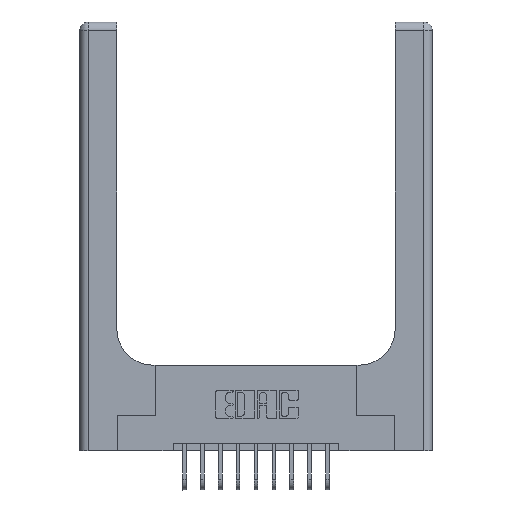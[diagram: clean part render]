
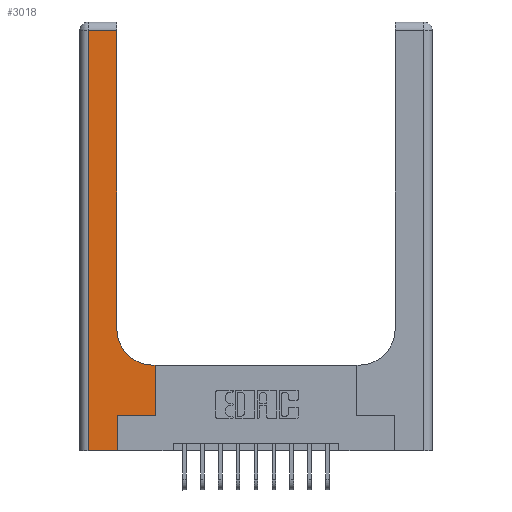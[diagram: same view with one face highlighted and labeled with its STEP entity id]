
A CAD part, top view. The second image highlights one B-rep face of the part: STEP entity #3018.
In plain terms, the highlighted planar face has unit normal (0, 0, 1).
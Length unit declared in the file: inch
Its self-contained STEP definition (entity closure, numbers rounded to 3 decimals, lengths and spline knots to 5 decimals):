
#405 = LINE ( 'NONE', #14723, #9553 ) ;
#573 = DIRECTION ( 'NONE',  ( 0., 0., -1. ) ) ;
#615 = AXIS2_PLACEMENT_3D ( 'NONE', #7003, #573, #727 ) ;
#727 = DIRECTION ( 'NONE',  ( 1., 0., 0. ) ) ;
#802 = DIRECTION ( 'NONE',  ( 0., 0., -1. ) ) ;
#1181 = EDGE_CURVE ( 'NONE', #4048, #1853, #5839, .T. ) ;
#1262 = LINE ( 'NONE', #6699, #10371 ) ;
#1853 = VERTEX_POINT ( 'NONE', #13303 ) ;
#1867 = CARTESIAN_POINT ( 'NONE',  ( 0., 2.94, 0.37 ) ) ;
#1928 = DIRECTION ( 'NONE',  ( 1., 0., 0. ) ) ;
#2001 = EDGE_CURVE ( 'NONE', #9961, #12800, #8169, .T. ) ;
#2038 = VECTOR ( 'NONE', #13661, 39.37008 ) ;
#2502 = EDGE_CURVE ( 'NONE', #14931, #10751, #4890, .T. ) ;
#2544 = ORIENTED_EDGE ( 'NONE', *, *, #8270, .T. ) ;
#2591 = VERTEX_POINT ( 'NONE', #9210 ) ;
#2770 = LINE ( 'NONE', #3832, #11812 ) ;
#3018 = ADVANCED_FACE ( 'NONE', ( #6888 ), #6785, .F. ) ;
#3832 = CARTESIAN_POINT ( 'NONE',  ( 0.06, 3., 0.37 ) ) ;
#4048 = VERTEX_POINT ( 'NONE', #14585 ) ;
#4334 = CARTESIAN_POINT ( 'NONE',  ( 0.265, 0.25, 0.37 ) ) ;
#4401 = VECTOR ( 'NONE', #9011, 39.37008 ) ;
#4403 = CARTESIAN_POINT ( 'NONE',  ( 0., 3., 0.37 ) ) ;
#4890 = LINE ( 'NONE', #1867, #2038 ) ;
#5071 = VECTOR ( 'NONE', #6713, 39.37008 ) ;
#5186 = LINE ( 'NONE', #11424, #14109 ) ;
#5289 = LINE ( 'NONE', #6339, #11146 ) ;
#5428 = VERTEX_POINT ( 'NONE', #4334 ) ;
#5543 = DIRECTION ( 'NONE',  ( 1., 0., 0. ) ) ;
#5839 = CIRCLE ( 'NONE', #615, 0.25 ) ;
#5949 = EDGE_CURVE ( 'NONE', #12800, #4048, #10299, .T. ) ;
#6060 = CARTESIAN_POINT ( 'NONE',  ( 0.528, 0.6, 0.37 ) ) ;
#6246 = DIRECTION ( 'NONE',  ( 0., -1., 0. ) ) ;
#6339 = CARTESIAN_POINT ( 'NONE',  ( 0.26, 3., 0.37 ) ) ;
#6534 = EDGE_CURVE ( 'NONE', #2591, #5428, #405, .T. ) ;
#6549 = DIRECTION ( 'NONE',  ( 0., 1., 0. ) ) ;
#6699 = CARTESIAN_POINT ( 'NONE',  ( 0., 0., 0.37 ) ) ;
#6713 = DIRECTION ( 'NONE',  ( 0., 1., 0. ) ) ;
#6785 = PLANE ( 'NONE',  #11084 ) ;
#6847 = CARTESIAN_POINT ( 'NONE',  ( 0.06, 2.94, 0.37 ) ) ;
#6888 = FACE_OUTER_BOUND ( 'NONE', #12402, .T. ) ;
#7003 = CARTESIAN_POINT ( 'NONE',  ( 0.51, 0.85, 0.37 ) ) ;
#8169 = LINE ( 'NONE', #11322, #5071 ) ;
#8270 = EDGE_CURVE ( 'NONE', #1853, #14931, #5289, .T. ) ;
#8445 = ORIENTED_EDGE ( 'NONE', *, *, #2502, .T. ) ;
#8645 = ORIENTED_EDGE ( 'NONE', *, *, #11023, .T. ) ;
#8878 = ORIENTED_EDGE ( 'NONE', *, *, #10664, .T. ) ;
#8997 = ORIENTED_EDGE ( 'NONE', *, *, #6534, .T. ) ;
#9011 = DIRECTION ( 'NONE',  ( -1., 0., 0. ) ) ;
#9144 = DIRECTION ( 'NONE',  ( -1., 0., 0. ) ) ;
#9169 = ORIENTED_EDGE ( 'NONE', *, *, #12541, .T. ) ;
#9210 = CARTESIAN_POINT ( 'NONE',  ( 0.265, 0., 0.37 ) ) ;
#9333 = ORIENTED_EDGE ( 'NONE', *, *, #2001, .T. ) ;
#9464 = ORIENTED_EDGE ( 'NONE', *, *, #5949, .T. ) ;
#9472 = CARTESIAN_POINT ( 'NONE',  ( 0.26, 2.94, 0.37 ) ) ;
#9553 = VECTOR ( 'NONE', #6549, 39.37008 ) ;
#9661 = CARTESIAN_POINT ( 'NONE',  ( 0.06, 0., 0.37 ) ) ;
#9961 = VERTEX_POINT ( 'NONE', #10121 ) ;
#9967 = ORIENTED_EDGE ( 'NONE', *, *, #1181, .T. ) ;
#10121 = CARTESIAN_POINT ( 'NONE',  ( 0.528, 0.25, 0.37 ) ) ;
#10200 = CARTESIAN_POINT ( 'NONE',  ( 0.26, 0.6, 0.37 ) ) ;
#10299 = LINE ( 'NONE', #10200, #4401 ) ;
#10371 = VECTOR ( 'NONE', #1928, 39.37008 ) ;
#10664 = EDGE_CURVE ( 'NONE', #11641, #2591, #1262, .T. ) ;
#10751 = VERTEX_POINT ( 'NONE', #6847 ) ;
#11023 = EDGE_CURVE ( 'NONE', #10751, #11641, #2770, .T. ) ;
#11084 = AXIS2_PLACEMENT_3D ( 'NONE', #4403, #802, #9144 ) ;
#11146 = VECTOR ( 'NONE', #14447, 39.37008 ) ;
#11322 = CARTESIAN_POINT ( 'NONE',  ( 0.528, 0.25, 0.37 ) ) ;
#11424 = CARTESIAN_POINT ( 'NONE',  ( 0.265, 0.25, 0.37 ) ) ;
#11641 = VERTEX_POINT ( 'NONE', #9661 ) ;
#11812 = VECTOR ( 'NONE', #6246, 39.37008 ) ;
#12402 = EDGE_LOOP ( 'NONE', ( #2544, #8445, #8645, #8878, #8997, #9169, #9333, #9464, #9967 ) ) ;
#12541 = EDGE_CURVE ( 'NONE', #5428, #9961, #5186, .T. ) ;
#12800 = VERTEX_POINT ( 'NONE', #6060 ) ;
#13303 = CARTESIAN_POINT ( 'NONE',  ( 0.26, 0.85, 0.37 ) ) ;
#13661 = DIRECTION ( 'NONE',  ( -1., 0., 0. ) ) ;
#14109 = VECTOR ( 'NONE', #5543, 39.37008 ) ;
#14447 = DIRECTION ( 'NONE',  ( 0., 1., 0. ) ) ;
#14585 = CARTESIAN_POINT ( 'NONE',  ( 0.51, 0.6, 0.37 ) ) ;
#14723 = CARTESIAN_POINT ( 'NONE',  ( 0.265, 0., 0.37 ) ) ;
#14931 = VERTEX_POINT ( 'NONE', #9472 ) ;
